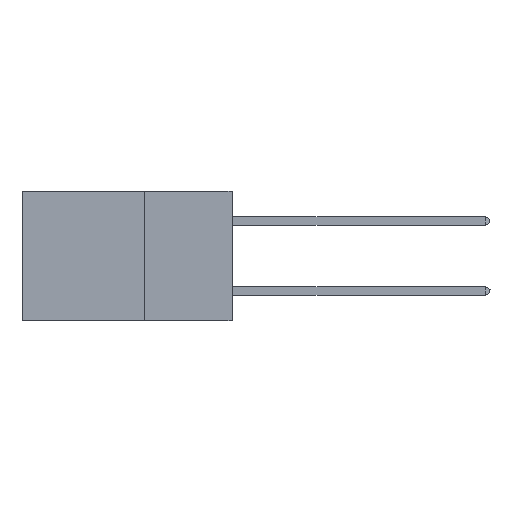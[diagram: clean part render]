
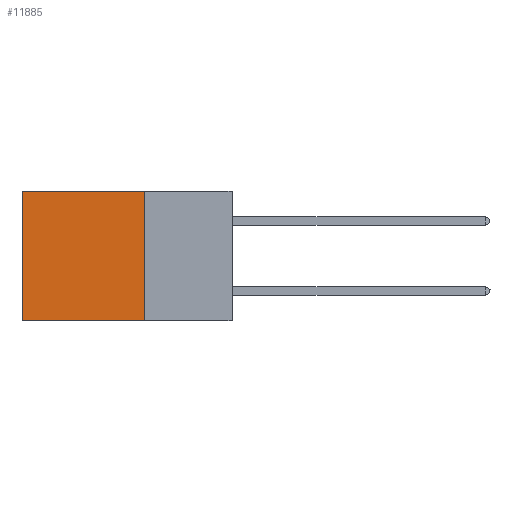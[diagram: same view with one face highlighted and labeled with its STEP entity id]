
A CAD part, left-side view. The second image highlights one B-rep face of the part: STEP entity #11885.
In plain terms, the highlighted planar face has unit normal (-1, 0, 0).
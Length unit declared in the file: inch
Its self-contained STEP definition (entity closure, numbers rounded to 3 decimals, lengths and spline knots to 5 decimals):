
#869 = ORIENTED_EDGE ( 'NONE', *, *, #14186, .F. ) ;
#983 = VERTEX_POINT ( 'NONE', #8884 ) ;
#1105 = CARTESIAN_POINT ( 'NONE',  ( 0.2875, 0.6, 0. ) ) ;
#1472 = LINE ( 'NONE', #4760, #8453 ) ;
#2665 = PLANE ( 'NONE',  #15996 ) ;
#2867 = EDGE_CURVE ( 'NONE', #6362, #983, #16647, .T. ) ;
#3010 = DIRECTION ( 'NONE',  ( 0., 0., -1. ) ) ;
#3299 = FACE_OUTER_BOUND ( 'NONE', #4767, .T. ) ;
#3351 = DIRECTION ( 'NONE',  ( 0., 1., 0. ) ) ;
#4185 = VERTEX_POINT ( 'NONE', #14504 ) ;
#4760 = CARTESIAN_POINT ( 'NONE',  ( 0.2875, 0.25, -0.37 ) ) ;
#4767 = EDGE_LOOP ( 'NONE', ( #12762, #869, #7905, #11681 ) ) ;
#6362 = VERTEX_POINT ( 'NONE', #12522 ) ;
#6878 = DIRECTION ( 'NONE',  ( 0., 0., -1. ) ) ;
#7072 = VECTOR ( 'NONE', #3010, 39.37008 ) ;
#7905 = ORIENTED_EDGE ( 'NONE', *, *, #2867, .F. ) ;
#8453 = VECTOR ( 'NONE', #3351, 39.37008 ) ;
#8884 = CARTESIAN_POINT ( 'NONE',  ( 0.2875, 0.25, -0.37 ) ) ;
#9690 = LINE ( 'NONE', #16580, #10146 ) ;
#9722 = DIRECTION ( 'NONE',  ( 0., 1., 0. ) ) ;
#10065 = EDGE_CURVE ( 'NONE', #13153, #4185, #14453, .T. ) ;
#10146 = VECTOR ( 'NONE', #9722, 39.37008 ) ;
#11567 = CARTESIAN_POINT ( 'NONE',  ( 0.2875, 0.25, 0. ) ) ;
#11681 = ORIENTED_EDGE ( 'NONE', *, *, #17122, .T. ) ;
#11885 = ADVANCED_FACE ( 'NONE', ( #3299 ), #2665, .F. ) ;
#12522 = CARTESIAN_POINT ( 'NONE',  ( 0.2875, 0.25, 0. ) ) ;
#12762 = ORIENTED_EDGE ( 'NONE', *, *, #10065, .T. ) ;
#13006 = DIRECTION ( 'NONE',  ( 0., 0., -1. ) ) ;
#13034 = VECTOR ( 'NONE', #13006, 39.37008 ) ;
#13153 = VERTEX_POINT ( 'NONE', #1105 ) ;
#14186 = EDGE_CURVE ( 'NONE', #983, #4185, #1472, .T. ) ;
#14453 = LINE ( 'NONE', #15501, #7072 ) ;
#14504 = CARTESIAN_POINT ( 'NONE',  ( 0.2875, 0.6, -0.37 ) ) ;
#15019 = CARTESIAN_POINT ( 'NONE',  ( 0.2875, 0.25, 0. ) ) ;
#15190 = DIRECTION ( 'NONE',  ( 1., 0., 0. ) ) ;
#15501 = CARTESIAN_POINT ( 'NONE',  ( 0.2875, 0.6, 0. ) ) ;
#15996 = AXIS2_PLACEMENT_3D ( 'NONE', #15019, #15190, #6878 ) ;
#16580 = CARTESIAN_POINT ( 'NONE',  ( 0.2875, 0.25, 0. ) ) ;
#16647 = LINE ( 'NONE', #11567, #13034 ) ;
#17122 = EDGE_CURVE ( 'NONE', #6362, #13153, #9690, .T. ) ;
